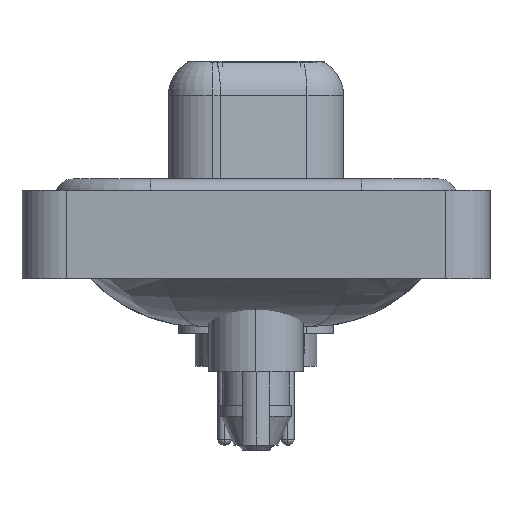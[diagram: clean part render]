
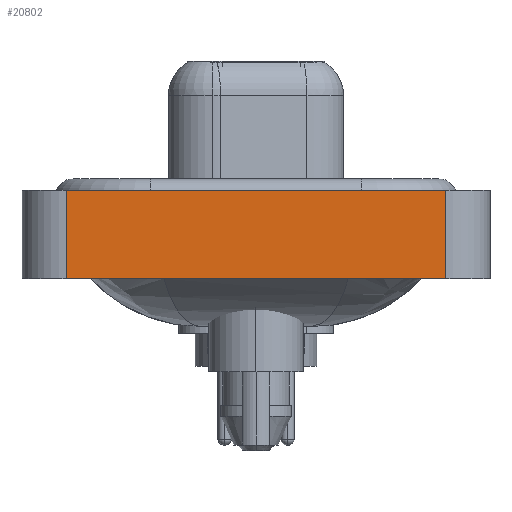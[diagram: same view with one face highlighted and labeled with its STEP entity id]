
A CAD part, left-side view. The second image highlights one B-rep face of the part: STEP entity #20802.
In plain terms, the highlighted planar face has unit normal (-1, 0, 0).
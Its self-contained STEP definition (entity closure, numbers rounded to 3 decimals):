
#76 = CARTESIAN_POINT ( 'NONE',  ( -7.35, 8.55, 0.4 ) ) ;
#1059 = LINE ( 'NONE', #15794, #12936 ) ;
#1551 = EDGE_CURVE ( 'NONE', #13163, #25082, #16219, .T. ) ;
#2001 = EDGE_CURVE ( 'NONE', #16168, #23580, #1059, .T. ) ;
#3249 = DIRECTION ( 'NONE',  ( 0., 0., 1. ) ) ;
#3288 = DIRECTION ( 'NONE',  ( 0., -1., 0. ) ) ;
#3548 = CARTESIAN_POINT ( 'NONE',  ( -7.35, -8.55, 0.4 ) ) ;
#4048 = EDGE_CURVE ( 'NONE', #25082, #23580, #21362, .T. ) ;
#4419 = CARTESIAN_POINT ( 'NONE',  ( -7.35, -8.55, 0.4 ) ) ;
#5404 = ORIENTED_EDGE ( 'NONE', *, *, #4048, .F. ) ;
#6249 = CARTESIAN_POINT ( 'NONE',  ( -7.35, -8.55, -3.6 ) ) ;
#7079 = FACE_OUTER_BOUND ( 'NONE', #23955, .T. ) ;
#9279 = DIRECTION ( 'NONE',  ( -1., 0., 0. ) ) ;
#10087 = CARTESIAN_POINT ( 'NONE',  ( -7.35, 8.55, -3.6 ) ) ;
#11331 = PLANE ( 'NONE',  #26540 ) ;
#11761 = LINE ( 'NONE', #24028, #19005 ) ;
#12936 = VECTOR ( 'NONE', #23987, 1000. ) ;
#13163 = VERTEX_POINT ( 'NONE', #16513 ) ;
#14194 = ORIENTED_EDGE ( 'NONE', *, *, #15573, .T. ) ;
#15573 = EDGE_CURVE ( 'NONE', #13163, #16168, #11761, .T. ) ;
#15794 = CARTESIAN_POINT ( 'NONE',  ( -7.35, -8.55, -3.6 ) ) ;
#16168 = VERTEX_POINT ( 'NONE', #6249 ) ;
#16219 = LINE ( 'NONE', #10087, #16810 ) ;
#16513 = CARTESIAN_POINT ( 'NONE',  ( -7.35, 8.55, -3.6 ) ) ;
#16810 = VECTOR ( 'NONE', #18151, 1000. ) ;
#18151 = DIRECTION ( 'NONE',  ( 0., 0., 1. ) ) ;
#19005 = VECTOR ( 'NONE', #3288, 1000. ) ;
#19323 = DIRECTION ( 'NONE',  ( 0., -1., 0. ) ) ;
#20271 = ORIENTED_EDGE ( 'NONE', *, *, #2001, .T. ) ;
#20802 = ADVANCED_FACE ( 'NONE', ( #7079 ), #11331, .T. ) ;
#21362 = LINE ( 'NONE', #4419, #23843 ) ;
#23580 = VERTEX_POINT ( 'NONE', #3548 ) ;
#23776 = ORIENTED_EDGE ( 'NONE', *, *, #1551, .F. ) ;
#23843 = VECTOR ( 'NONE', #19323, 1000. ) ;
#23955 = EDGE_LOOP ( 'NONE', ( #20271, #5404, #23776, #14194 ) ) ;
#23987 = DIRECTION ( 'NONE',  ( 0., 0., 1. ) ) ;
#24028 = CARTESIAN_POINT ( 'NONE',  ( -7.35, -8.55, -3.6 ) ) ;
#25082 = VERTEX_POINT ( 'NONE', #76 ) ;
#25797 = CARTESIAN_POINT ( 'NONE',  ( -7.35, -8.55, -3.6 ) ) ;
#26540 = AXIS2_PLACEMENT_3D ( 'NONE', #25797, #9279, #3249 ) ;
